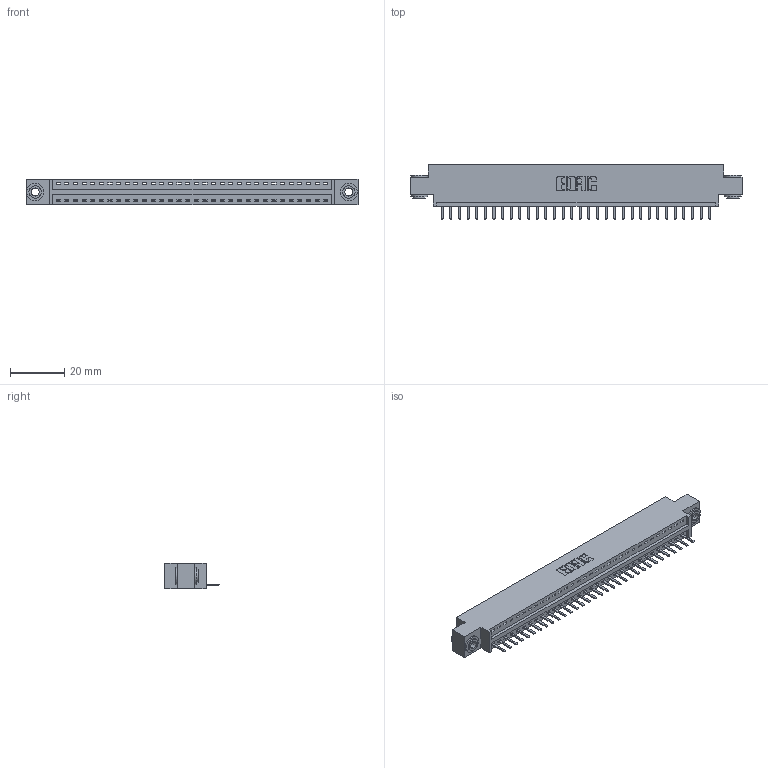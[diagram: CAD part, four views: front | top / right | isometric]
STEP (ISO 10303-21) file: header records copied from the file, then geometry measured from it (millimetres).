
FILE_DESCRIPTION (( 'STEP AP203' ), '1' );
FILE_NAME ('396-032-520-603.STEP', '2018-09-05T09:46:14', ( '' ), ( '' ), 'SwSTEP 2.0', 'SolidWorks 2016', '' );
FILE_SCHEMA (( 'CONFIG_CONTROL_DESIGN' ));
Length unit declared in the file: inch
Products named in the file (4): 346 Part_0.170 Offset - 0.156 Dia-TH; 345-292-001_345-293-120; 345-250-002_345-250-002-102; 396-032-520-603
Assembly tree (35 placements, depth 2):
  396-032-520-603
    346 Part_0.170 Offset - 0.156 Dia-TH
    345-292-001_345-293-120  x32
    345-250-002_345-250-002-102  x2
Bounding box: 122.17 x 20.02 x 9.4 mm (x, y, z)
Volume: 11398.6 mm3; surface area: 14211.1 mm2
Topology: 35 solids, 35 shells, 2148 faces, 6305 edges, 4114 vertices
Faces by surface type: plane 1434, cylinder 706, cone 8
Entity records: 22102 total; most frequent: CARTESIAN_POINT 3783, ORIENTED_EDGE 3730, DIRECTION 3367, EDGE_CURVE 1865, LINE 1577, VECTOR 1577, VERTEX_POINT 1238, AXIS2_PLACEMENT_3D 895
